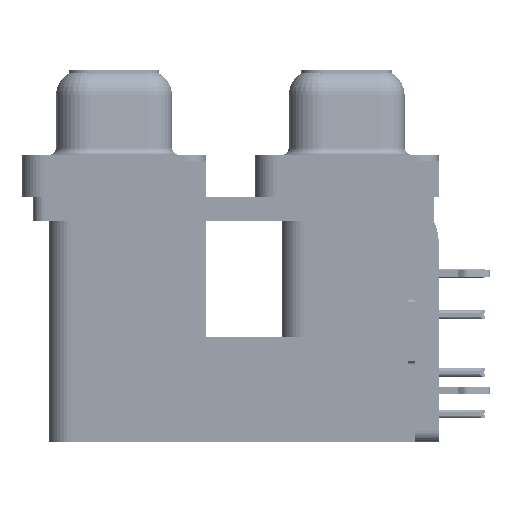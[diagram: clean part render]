
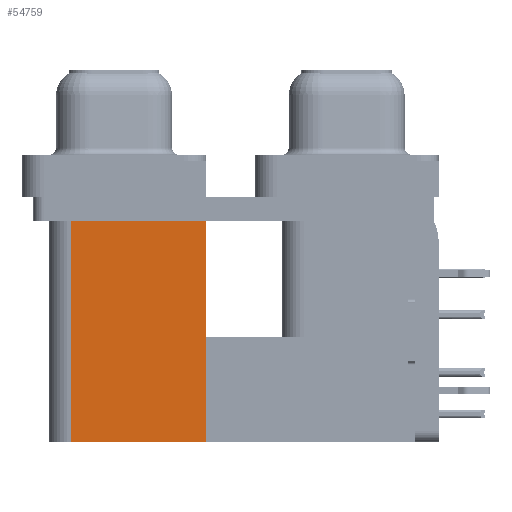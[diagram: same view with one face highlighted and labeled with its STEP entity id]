
A CAD part, left-side view. The second image highlights one B-rep face of the part: STEP entity #54759.
In plain terms, the highlighted planar face has unit normal (-1, 0, 0).
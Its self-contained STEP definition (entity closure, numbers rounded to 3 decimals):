
#651 = ORIENTED_EDGE ( 'NONE', *, *, #40976, .F. ) ;
#2876 = FACE_OUTER_BOUND ( 'NONE', #42631, .T. ) ;
#6459 = EDGE_CURVE ( 'NONE', #52068, #14833, #28215, .T. ) ;
#6807 = CARTESIAN_POINT ( 'NONE',  ( 3.7, 18.8, -2.5 ) ) ;
#7828 = VECTOR ( 'NONE', #47383, 1000. ) ;
#8704 = VERTEX_POINT ( 'NONE', #17564 ) ;
#9142 = CARTESIAN_POINT ( 'NONE',  ( 3.7, 9.6, -19.2 ) ) ;
#11095 = EDGE_CURVE ( 'NONE', #8704, #52068, #52804, .T. ) ;
#11976 = ORIENTED_EDGE ( 'NONE', *, *, #11095, .T. ) ;
#12163 = CARTESIAN_POINT ( 'NONE',  ( 3.7, 9.6, -19.2 ) ) ;
#14833 = VERTEX_POINT ( 'NONE', #6807 ) ;
#17228 = CARTESIAN_POINT ( 'NONE',  ( 3.7, 18.8, -19.2 ) ) ;
#17564 = CARTESIAN_POINT ( 'NONE',  ( 3.7, 9.6, -19.2 ) ) ;
#19354 = ORIENTED_EDGE ( 'NONE', *, *, #6459, .T. ) ;
#23002 = CARTESIAN_POINT ( 'NONE',  ( 3.7, 9.6, -19.2 ) ) ;
#25570 = VECTOR ( 'NONE', #44342, 1000. ) ;
#27119 = DIRECTION ( 'NONE',  ( 0., 1., 0. ) ) ;
#28157 = CARTESIAN_POINT ( 'NONE',  ( 3.7, 9.6, -2.5 ) ) ;
#28215 = LINE ( 'NONE', #43195, #47192 ) ;
#32482 = AXIS2_PLACEMENT_3D ( 'NONE', #12163, #61267, #27119 ) ;
#32524 = LINE ( 'NONE', #23002, #34461 ) ;
#34461 = VECTOR ( 'NONE', #52327, 1000. ) ;
#35480 = EDGE_CURVE ( 'NONE', #8704, #43307, #32524, .T. ) ;
#38114 = DIRECTION ( 'NONE',  ( 0., 1., 0. ) ) ;
#40976 = EDGE_CURVE ( 'NONE', #43307, #14833, #53331, .T. ) ;
#41757 = PLANE ( 'NONE',  #32482 ) ;
#42631 = EDGE_LOOP ( 'NONE', ( #19354, #651, #52763, #11976 ) ) ;
#43195 = CARTESIAN_POINT ( 'NONE',  ( 3.7, 9.6, -2.5 ) ) ;
#43307 = VERTEX_POINT ( 'NONE', #17228 ) ;
#44342 = DIRECTION ( 'NONE',  ( 0., 0., 1. ) ) ;
#47192 = VECTOR ( 'NONE', #38114, 1000. ) ;
#47383 = DIRECTION ( 'NONE',  ( 0., 0., 1. ) ) ;
#49152 = CARTESIAN_POINT ( 'NONE',  ( 3.7, 18.8, -19.2 ) ) ;
#52068 = VERTEX_POINT ( 'NONE', #28157 ) ;
#52327 = DIRECTION ( 'NONE',  ( 0., 1., 0. ) ) ;
#52763 = ORIENTED_EDGE ( 'NONE', *, *, #35480, .F. ) ;
#52804 = LINE ( 'NONE', #9142, #7828 ) ;
#53331 = LINE ( 'NONE', #49152, #25570 ) ;
#54759 = ADVANCED_FACE ( 'NONE', ( #2876 ), #41757, .F. ) ;
#61267 = DIRECTION ( 'NONE',  ( 1., 0., 0. ) ) ;
